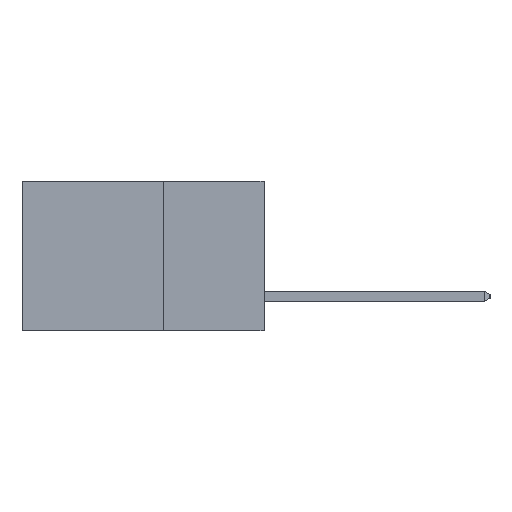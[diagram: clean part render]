
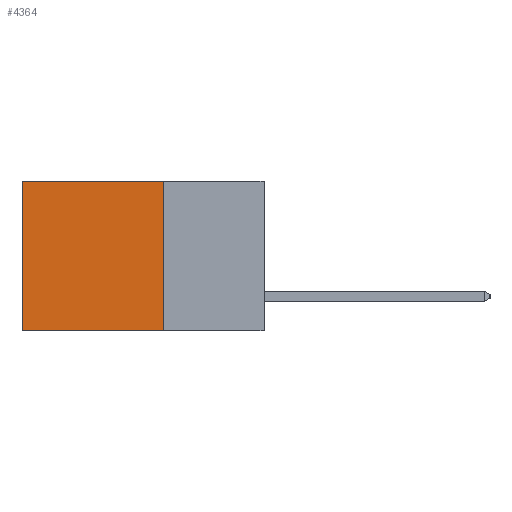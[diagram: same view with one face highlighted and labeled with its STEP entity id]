
A CAD part, left-side view. The second image highlights one B-rep face of the part: STEP entity #4364.
In plain terms, the highlighted planar face has unit normal (-1, 0, 0).
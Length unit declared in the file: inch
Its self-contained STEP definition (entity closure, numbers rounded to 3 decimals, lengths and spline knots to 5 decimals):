
#77 = CARTESIAN_POINT ( 'NONE',  ( 0.2615, 0.6, -0.37 ) ) ;
#331 = VERTEX_POINT ( 'NONE', #8701 ) ;
#479 = DIRECTION ( 'NONE',  ( 1., 0., 0. ) ) ;
#801 = CARTESIAN_POINT ( 'NONE',  ( 0.2615, 0.6, -0.37 ) ) ;
#1778 = FACE_OUTER_BOUND ( 'NONE', #6835, .T. ) ;
#1780 = ORIENTED_EDGE ( 'NONE', *, *, #4472, .T. ) ;
#1792 = ORIENTED_EDGE ( 'NONE', *, *, #7760, .F. ) ;
#1821 = ORIENTED_EDGE ( 'NONE', *, *, #11343, .F. ) ;
#1836 = ORIENTED_EDGE ( 'NONE', *, *, #7599, .T. ) ;
#2941 = VECTOR ( 'NONE', #9229, 39.37008 ) ;
#3424 = VERTEX_POINT ( 'NONE', #10817 ) ;
#3805 = CARTESIAN_POINT ( 'NONE',  ( 0.2615, 0.25, -0.37 ) ) ;
#3814 = VECTOR ( 'NONE', #9299, 39.37008 ) ;
#4364 = ADVANCED_FACE ( 'NONE', ( #1778 ), #11324, .F. ) ;
#4472 = EDGE_CURVE ( 'NONE', #331, #6053, #11605, .T. ) ;
#4642 = CARTESIAN_POINT ( 'NONE',  ( 0.2615, 0.25, -0.37 ) ) ;
#5029 = LINE ( 'NONE', #5654, #7152 ) ;
#5486 = VECTOR ( 'NONE', #7604, 39.37008 ) ;
#5498 = LINE ( 'NONE', #3805, #2941 ) ;
#5654 = CARTESIAN_POINT ( 'NONE',  ( 0.2615, 0.25, 0. ) ) ;
#6053 = VERTEX_POINT ( 'NONE', #77 ) ;
#6561 = DIRECTION ( 'NONE',  ( 0., 1., 0. ) ) ;
#6719 = CARTESIAN_POINT ( 'NONE',  ( 0.2615, 0.25, -0.37 ) ) ;
#6835 = EDGE_LOOP ( 'NONE', ( #1780, #1792, #1821, #1836 ) ) ;
#7152 = VECTOR ( 'NONE', #6561, 39.37008 ) ;
#7599 = EDGE_CURVE ( 'NONE', #3424, #331, #5029, .T. ) ;
#7604 = DIRECTION ( 'NONE',  ( 0., 0., -1. ) ) ;
#7760 = EDGE_CURVE ( 'NONE', #10160, #6053, #8397, .T. ) ;
#8397 = LINE ( 'NONE', #8488, #3814 ) ;
#8488 = CARTESIAN_POINT ( 'NONE',  ( 0.2615, 0.25, -0.37 ) ) ;
#8569 = AXIS2_PLACEMENT_3D ( 'NONE', #4642, #479, #10566 ) ;
#8701 = CARTESIAN_POINT ( 'NONE',  ( 0.2615, 0.6, 0. ) ) ;
#9229 = DIRECTION ( 'NONE',  ( 0., 0., -1. ) ) ;
#9299 = DIRECTION ( 'NONE',  ( 0., 1., 0. ) ) ;
#10160 = VERTEX_POINT ( 'NONE', #6719 ) ;
#10566 = DIRECTION ( 'NONE',  ( 0., 0., -1. ) ) ;
#10817 = CARTESIAN_POINT ( 'NONE',  ( 0.2615, 0.25, 0. ) ) ;
#11324 = PLANE ( 'NONE',  #8569 ) ;
#11343 = EDGE_CURVE ( 'NONE', #3424, #10160, #5498, .T. ) ;
#11605 = LINE ( 'NONE', #801, #5486 ) ;
